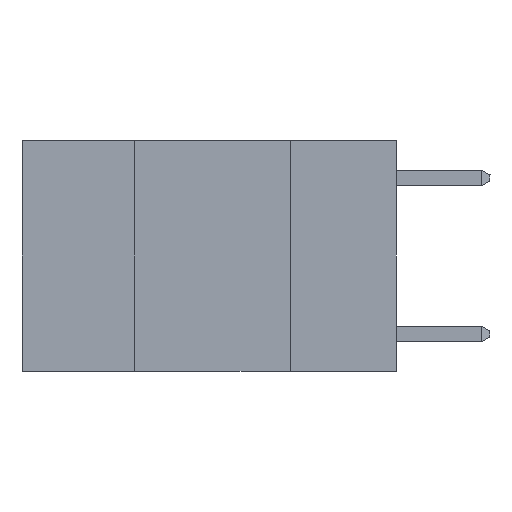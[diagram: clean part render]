
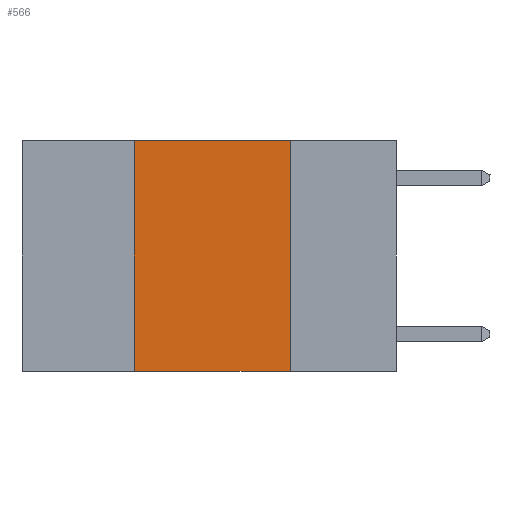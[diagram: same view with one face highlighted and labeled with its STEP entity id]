
A CAD part, left-side view. The second image highlights one B-rep face of the part: STEP entity #566.
In plain terms, the highlighted planar face has unit normal (-1, 0, 0).
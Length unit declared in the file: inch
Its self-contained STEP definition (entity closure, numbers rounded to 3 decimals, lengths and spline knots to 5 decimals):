
#33 = VERTEX_POINT ( 'NONE', #3342 ) ;
#128 = PLANE ( 'NONE',  #664 ) ;
#497 = CARTESIAN_POINT ( 'NONE',  ( 0., 0.6, 0. ) ) ;
#566 = ADVANCED_FACE ( 'NONE', ( #1363 ), #128, .F. ) ;
#664 = AXIS2_PLACEMENT_3D ( 'NONE', #497, #3922, #6587 ) ;
#1363 = FACE_OUTER_BOUND ( 'NONE', #9599, .T. ) ;
#2293 = CARTESIAN_POINT ( 'NONE',  ( 0., 0.17, 0. ) ) ;
#2383 = EDGE_CURVE ( 'NONE', #2980, #3143, #8795, .T. ) ;
#2405 = EDGE_CURVE ( 'NONE', #2980, #33, #8707, .T. ) ;
#2415 = EDGE_CURVE ( 'NONE', #3809, #3143, #8635, .T. ) ;
#2552 = EDGE_CURVE ( 'NONE', #33, #3809, #8044, .T. ) ;
#2657 = ORIENTED_EDGE ( 'NONE', *, *, #2405, .F. ) ;
#2980 = VERTEX_POINT ( 'NONE', #8762 ) ;
#3143 = VERTEX_POINT ( 'NONE', #7718 ) ;
#3342 = CARTESIAN_POINT ( 'NONE',  ( 0., 0.42, 0. ) ) ;
#3809 = VERTEX_POINT ( 'NONE', #2293 ) ;
#3922 = DIRECTION ( 'NONE',  ( 1., 0., 0. ) ) ;
#4559 = DIRECTION ( 'NONE',  ( 0., -1., 0. ) ) ;
#4707 = CARTESIAN_POINT ( 'NONE',  ( 0., 0.6, 0. ) ) ;
#6587 = DIRECTION ( 'NONE',  ( 0., 0., -1. ) ) ;
#6809 = DIRECTION ( 'NONE',  ( 0., 0., -1. ) ) ;
#6881 = CARTESIAN_POINT ( 'NONE',  ( 0., 0.17, 0. ) ) ;
#7040 = CARTESIAN_POINT ( 'NONE',  ( 0., 0.42, 0. ) ) ;
#7136 = DIRECTION ( 'NONE',  ( 0., 0., 1. ) ) ;
#7245 = CARTESIAN_POINT ( 'NONE',  ( 0., 0.6, -0.37 ) ) ;
#7328 = DIRECTION ( 'NONE',  ( 0., -1., 0. ) ) ;
#7718 = CARTESIAN_POINT ( 'NONE',  ( 0., 0.17, -0.37 ) ) ;
#7983 = VECTOR ( 'NONE', #4559, 39.37008 ) ;
#8044 = LINE ( 'NONE', #4707, #7983 ) ;
#8252 = ORIENTED_EDGE ( 'NONE', *, *, #2415, .F. ) ;
#8378 = ORIENTED_EDGE ( 'NONE', *, *, #2552, .F. ) ;
#8418 = ORIENTED_EDGE ( 'NONE', *, *, #2383, .T. ) ;
#8631 = VECTOR ( 'NONE', #6809, 39.37008 ) ;
#8635 = LINE ( 'NONE', #6881, #8631 ) ;
#8645 = VECTOR ( 'NONE', #7136, 39.37008 ) ;
#8707 = LINE ( 'NONE', #7040, #8645 ) ;
#8735 = VECTOR ( 'NONE', #7328, 39.37008 ) ;
#8762 = CARTESIAN_POINT ( 'NONE',  ( 0., 0.42, -0.37 ) ) ;
#8795 = LINE ( 'NONE', #7245, #8735 ) ;
#9599 = EDGE_LOOP ( 'NONE', ( #8252, #8378, #2657, #8418 ) ) ;
